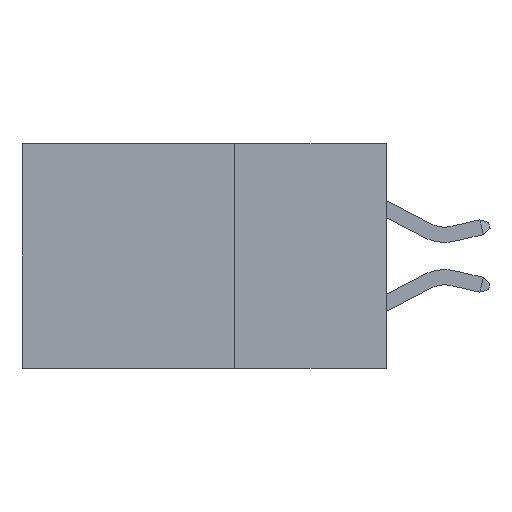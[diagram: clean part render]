
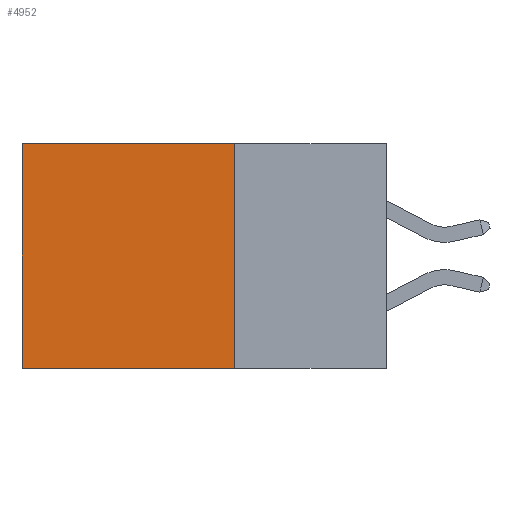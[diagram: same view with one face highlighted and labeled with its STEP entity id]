
A CAD part, left-side view. The second image highlights one B-rep face of the part: STEP entity #4952.
In plain terms, the highlighted planar face has unit normal (-1, 0, 0).
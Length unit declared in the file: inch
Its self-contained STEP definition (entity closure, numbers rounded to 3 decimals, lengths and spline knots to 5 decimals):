
#649 = DIRECTION ( 'NONE',  ( 0., 1., 0. ) ) ;
#1309 = LINE ( 'NONE', #1957, #6277 ) ;
#1457 = LINE ( 'NONE', #11959, #11330 ) ;
#1556 = VECTOR ( 'NONE', #7815, 39.37008 ) ;
#1738 = CARTESIAN_POINT ( 'NONE',  ( 0.298, 0.6, 0. ) ) ;
#1957 = CARTESIAN_POINT ( 'NONE',  ( 0.298, 0.6, 0. ) ) ;
#2311 = FACE_OUTER_BOUND ( 'NONE', #11259, .T. ) ;
#2662 = LINE ( 'NONE', #9458, #7347 ) ;
#2938 = DIRECTION ( 'NONE',  ( 0., 0., -1. ) ) ;
#4012 = AXIS2_PLACEMENT_3D ( 'NONE', #7771, #9584, #9552 ) ;
#4502 = LINE ( 'NONE', #7857, #1556 ) ;
#4569 = ORIENTED_EDGE ( 'NONE', *, *, #7134, .F. ) ;
#4902 = ORIENTED_EDGE ( 'NONE', *, *, #12596, .T. ) ;
#4952 = ADVANCED_FACE ( 'NONE', ( #2311 ), #7656, .F. ) ;
#6277 = VECTOR ( 'NONE', #2938, 39.37008 ) ;
#6603 = CARTESIAN_POINT ( 'NONE',  ( 0.298, 0.6, -0.37 ) ) ;
#7134 = EDGE_CURVE ( 'NONE', #10447, #8917, #4502, .T. ) ;
#7347 = VECTOR ( 'NONE', #649, 39.37008 ) ;
#7656 = PLANE ( 'NONE',  #4012 ) ;
#7771 = CARTESIAN_POINT ( 'NONE',  ( 0.298, 0.25, 0. ) ) ;
#7815 = DIRECTION ( 'NONE',  ( 0., 0., -1. ) ) ;
#7857 = CARTESIAN_POINT ( 'NONE',  ( 0.298, 0.25, 0. ) ) ;
#8917 = VERTEX_POINT ( 'NONE', #12427 ) ;
#9458 = CARTESIAN_POINT ( 'NONE',  ( 0.298, 0.25, 0. ) ) ;
#9492 = ORIENTED_EDGE ( 'NONE', *, *, #9834, .T. ) ;
#9552 = DIRECTION ( 'NONE',  ( 0., 0., -1. ) ) ;
#9584 = DIRECTION ( 'NONE',  ( 1., 0., 0. ) ) ;
#9834 = EDGE_CURVE ( 'NONE', #12689, #10659, #1309, .T. ) ;
#10447 = VERTEX_POINT ( 'NONE', #12154 ) ;
#10659 = VERTEX_POINT ( 'NONE', #6603 ) ;
#11259 = EDGE_LOOP ( 'NONE', ( #9492, #12143, #4569, #4902 ) ) ;
#11330 = VECTOR ( 'NONE', #11912, 39.37008 ) ;
#11912 = DIRECTION ( 'NONE',  ( 0., 1., 0. ) ) ;
#11959 = CARTESIAN_POINT ( 'NONE',  ( 0.298, 0.25, -0.37 ) ) ;
#12143 = ORIENTED_EDGE ( 'NONE', *, *, #12258, .F. ) ;
#12154 = CARTESIAN_POINT ( 'NONE',  ( 0.298, 0.25, 0. ) ) ;
#12258 = EDGE_CURVE ( 'NONE', #8917, #10659, #1457, .T. ) ;
#12427 = CARTESIAN_POINT ( 'NONE',  ( 0.298, 0.25, -0.37 ) ) ;
#12596 = EDGE_CURVE ( 'NONE', #10447, #12689, #2662, .T. ) ;
#12689 = VERTEX_POINT ( 'NONE', #1738 ) ;
